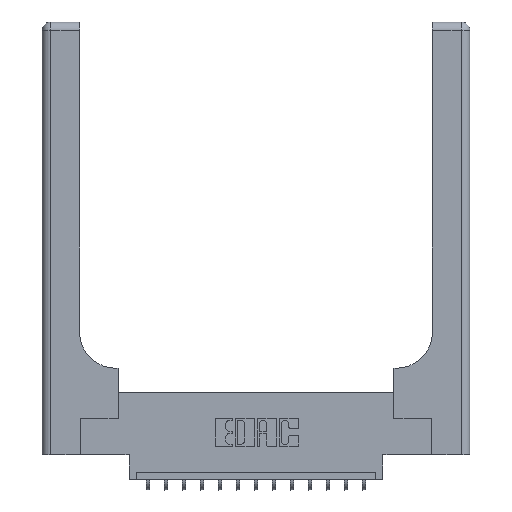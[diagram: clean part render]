
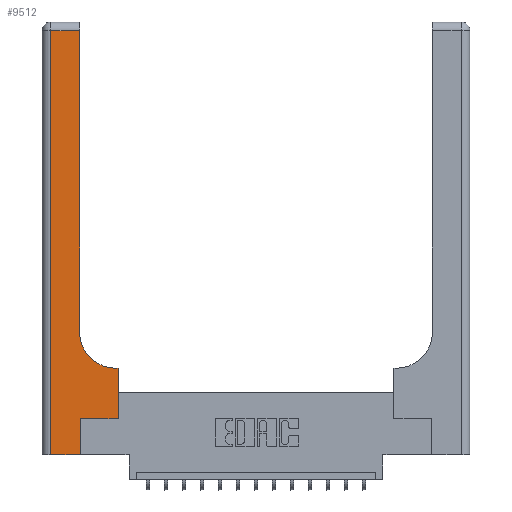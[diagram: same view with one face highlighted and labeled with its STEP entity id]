
A CAD part, top view. The second image highlights one B-rep face of the part: STEP entity #9512.
In plain terms, the highlighted planar face has unit normal (0, 0, 1).
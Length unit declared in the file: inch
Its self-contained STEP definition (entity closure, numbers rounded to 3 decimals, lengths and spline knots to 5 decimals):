
#588 = DIRECTION ( 'NONE',  ( 1., 0., 0. ) ) ;
#877 = CARTESIAN_POINT ( 'NONE',  ( 0.26, 2.94, 0.37 ) ) ;
#933 = LINE ( 'NONE', #1625, #4391 ) ;
#1267 = ORIENTED_EDGE ( 'NONE', *, *, #9071, .T. ) ;
#1358 = CARTESIAN_POINT ( 'NONE',  ( 0.265, 0., 0.37 ) ) ;
#1432 = EDGE_CURVE ( 'NONE', #9717, #4064, #7307, .T. ) ;
#1498 = CARTESIAN_POINT ( 'NONE',  ( 0.06, 0., 0.37 ) ) ;
#1590 = VERTEX_POINT ( 'NONE', #1498 ) ;
#1625 = CARTESIAN_POINT ( 'NONE',  ( 0.26, 3., 0.37 ) ) ;
#1792 = ORIENTED_EDGE ( 'NONE', *, *, #1432, .T. ) ;
#1840 = AXIS2_PLACEMENT_3D ( 'NONE', #10098, #10036, #9916 ) ;
#1881 = FACE_OUTER_BOUND ( 'NONE', #4063, .T. ) ;
#2213 = ORIENTED_EDGE ( 'NONE', *, *, #4671, .T. ) ;
#2317 = EDGE_CURVE ( 'NONE', #4064, #4230, #933, .T. ) ;
#2458 = EDGE_CURVE ( 'NONE', #6587, #3358, #16875, .T. ) ;
#3358 = VERTEX_POINT ( 'NONE', #8402 ) ;
#3988 = VECTOR ( 'NONE', #7088, 39.37008 ) ;
#4063 = EDGE_LOOP ( 'NONE', ( #12707, #9769, #9270, #12245, #14754, #12283, #1267, #2213, #1792 ) ) ;
#4064 = VERTEX_POINT ( 'NONE', #15217 ) ;
#4092 = LINE ( 'NONE', #1358, #7632 ) ;
#4230 = VERTEX_POINT ( 'NONE', #877 ) ;
#4391 = VECTOR ( 'NONE', #15046, 39.37008 ) ;
#4506 = PLANE ( 'NONE',  #8774 ) ;
#4671 = EDGE_CURVE ( 'NONE', #15786, #9717, #6401, .T. ) ;
#5853 = DIRECTION ( 'NONE',  ( 0., 0., -1. ) ) ;
#6360 = DIRECTION ( 'NONE',  ( -1., 0., 0. ) ) ;
#6401 = LINE ( 'NONE', #16962, #13090 ) ;
#6587 = VERTEX_POINT ( 'NONE', #13099 ) ;
#6738 = EDGE_CURVE ( 'NONE', #16952, #6587, #4092, .T. ) ;
#6991 = CARTESIAN_POINT ( 'NONE',  ( 0.528, 0.6, 0.37 ) ) ;
#7026 = VECTOR ( 'NONE', #14173, 39.37008 ) ;
#7088 = DIRECTION ( 'NONE',  ( 0., -1., 0. ) ) ;
#7178 = EDGE_CURVE ( 'NONE', #4230, #15476, #11604, .T. ) ;
#7307 = CIRCLE ( 'NONE', #1840, 0.25 ) ;
#7615 = VECTOR ( 'NONE', #6360, 39.37008 ) ;
#7632 = VECTOR ( 'NONE', #9397, 39.37008 ) ;
#8402 = CARTESIAN_POINT ( 'NONE',  ( 0.528, 0.25, 0.37 ) ) ;
#8653 = CARTESIAN_POINT ( 'NONE',  ( 0.528, 0.25, 0.37 ) ) ;
#8774 = AXIS2_PLACEMENT_3D ( 'NONE', #9747, #5853, #15185 ) ;
#9028 = CARTESIAN_POINT ( 'NONE',  ( 0., 2.94, 0.37 ) ) ;
#9071 = EDGE_CURVE ( 'NONE', #3358, #15786, #9461, .T. ) ;
#9270 = ORIENTED_EDGE ( 'NONE', *, *, #10864, .T. ) ;
#9397 = DIRECTION ( 'NONE',  ( 0., 1., 0. ) ) ;
#9461 = LINE ( 'NONE', #8653, #9875 ) ;
#9512 = ADVANCED_FACE ( 'NONE', ( #1881 ), #4506, .F. ) ;
#9717 = VERTEX_POINT ( 'NONE', #12967 ) ;
#9747 = CARTESIAN_POINT ( 'NONE',  ( 0., 3., 0.37 ) ) ;
#9769 = ORIENTED_EDGE ( 'NONE', *, *, #7178, .T. ) ;
#9875 = VECTOR ( 'NONE', #13923, 39.37008 ) ;
#9916 = DIRECTION ( 'NONE',  ( 1., 0., 0. ) ) ;
#10036 = DIRECTION ( 'NONE',  ( 0., 0., -1. ) ) ;
#10098 = CARTESIAN_POINT ( 'NONE',  ( 0.51, 0.85, 0.37 ) ) ;
#10226 = VECTOR ( 'NONE', #588, 39.37008 ) ;
#10582 = LINE ( 'NONE', #16691, #7026 ) ;
#10864 = EDGE_CURVE ( 'NONE', #15476, #1590, #11506, .T. ) ;
#11506 = LINE ( 'NONE', #12422, #3988 ) ;
#11604 = LINE ( 'NONE', #9028, #7615 ) ;
#11707 = DIRECTION ( 'NONE',  ( -1., 0., 0. ) ) ;
#12245 = ORIENTED_EDGE ( 'NONE', *, *, #13862, .T. ) ;
#12283 = ORIENTED_EDGE ( 'NONE', *, *, #2458, .T. ) ;
#12422 = CARTESIAN_POINT ( 'NONE',  ( 0.06, 3., 0.37 ) ) ;
#12707 = ORIENTED_EDGE ( 'NONE', *, *, #2317, .T. ) ;
#12796 = CARTESIAN_POINT ( 'NONE',  ( 0.06, 2.94, 0.37 ) ) ;
#12967 = CARTESIAN_POINT ( 'NONE',  ( 0.51, 0.6, 0.37 ) ) ;
#13090 = VECTOR ( 'NONE', #11707, 39.37008 ) ;
#13099 = CARTESIAN_POINT ( 'NONE',  ( 0.265, 0.25, 0.37 ) ) ;
#13862 = EDGE_CURVE ( 'NONE', #1590, #16952, #10582, .T. ) ;
#13923 = DIRECTION ( 'NONE',  ( 0., 1., 0. ) ) ;
#13972 = CARTESIAN_POINT ( 'NONE',  ( 0.265, 0., 0.37 ) ) ;
#14173 = DIRECTION ( 'NONE',  ( 1., 0., 0. ) ) ;
#14754 = ORIENTED_EDGE ( 'NONE', *, *, #6738, .T. ) ;
#15046 = DIRECTION ( 'NONE',  ( 0., 1., 0. ) ) ;
#15185 = DIRECTION ( 'NONE',  ( -1., 0., 0. ) ) ;
#15217 = CARTESIAN_POINT ( 'NONE',  ( 0.26, 0.85, 0.37 ) ) ;
#15476 = VERTEX_POINT ( 'NONE', #12796 ) ;
#15786 = VERTEX_POINT ( 'NONE', #6991 ) ;
#16681 = CARTESIAN_POINT ( 'NONE',  ( 0.265, 0.25, 0.37 ) ) ;
#16691 = CARTESIAN_POINT ( 'NONE',  ( 0., 0., 0.37 ) ) ;
#16875 = LINE ( 'NONE', #16681, #10226 ) ;
#16952 = VERTEX_POINT ( 'NONE', #13972 ) ;
#16962 = CARTESIAN_POINT ( 'NONE',  ( 0.26, 0.6, 0.37 ) ) ;
